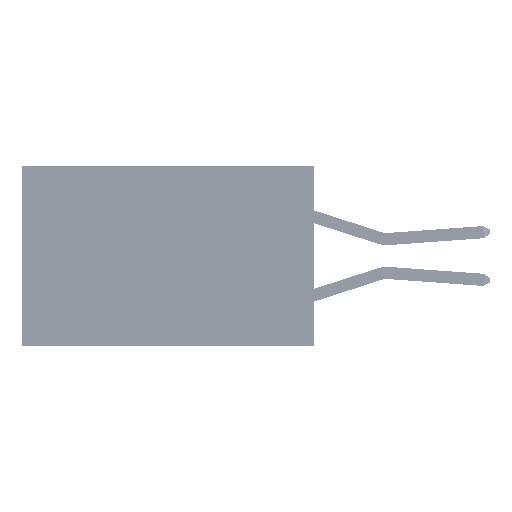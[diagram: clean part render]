
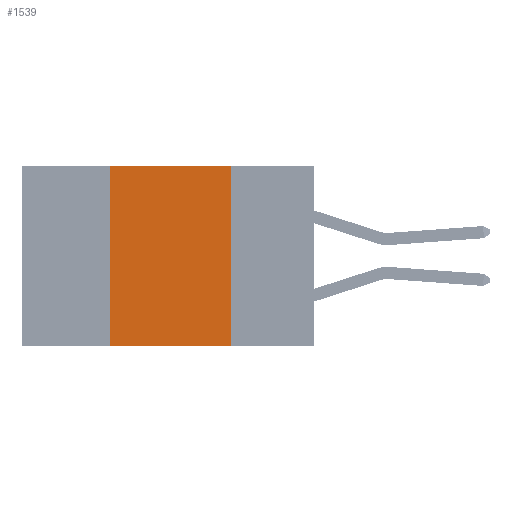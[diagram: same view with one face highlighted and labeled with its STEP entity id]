
A CAD part, left-side view. The second image highlights one B-rep face of the part: STEP entity #1539.
In plain terms, the highlighted planar face has unit normal (-1, 0, 0).
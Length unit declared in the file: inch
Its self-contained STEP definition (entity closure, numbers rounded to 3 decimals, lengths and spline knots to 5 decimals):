
#445 = CARTESIAN_POINT ( 'NONE',  ( 0., 0.42, -0.37 ) ) ;
#986 = DIRECTION ( 'NONE',  ( 0., 0., -1. ) ) ;
#1539 = ADVANCED_FACE ( 'NONE', ( #30907 ), #30218, .F. ) ;
#2058 = DIRECTION ( 'NONE',  ( 0., 0., -1. ) ) ;
#2326 = EDGE_CURVE ( 'NONE', #33802, #17893, #8206, .T. ) ;
#2948 = ORIENTED_EDGE ( 'NONE', *, *, #32629, .T. ) ;
#3927 = EDGE_LOOP ( 'NONE', ( #23682, #7659, #36213, #2948 ) ) ;
#5360 = LINE ( 'NONE', #33270, #23495 ) ;
#5584 = VECTOR ( 'NONE', #986, 39.37008 ) ;
#6009 = CARTESIAN_POINT ( 'NONE',  ( 0., 0.6, 0. ) ) ;
#6398 = VECTOR ( 'NONE', #20440, 39.37008 ) ;
#7060 = CARTESIAN_POINT ( 'NONE',  ( 0., 0.17, -0.37 ) ) ;
#7659 = ORIENTED_EDGE ( 'NONE', *, *, #41234, .F. ) ;
#8206 = LINE ( 'NONE', #43812, #5584 ) ;
#10143 = LINE ( 'NONE', #28269, #23420 ) ;
#10599 = DIRECTION ( 'NONE',  ( 0., 0., 1. ) ) ;
#12157 = VERTEX_POINT ( 'NONE', #445 ) ;
#16068 = DIRECTION ( 'NONE',  ( 0., -1., 0. ) ) ;
#17893 = VERTEX_POINT ( 'NONE', #7060 ) ;
#20440 = DIRECTION ( 'NONE',  ( 0., -1., 0. ) ) ;
#23420 = VECTOR ( 'NONE', #10599, 39.37008 ) ;
#23495 = VECTOR ( 'NONE', #16068, 39.37008 ) ;
#23682 = ORIENTED_EDGE ( 'NONE', *, *, #2326, .F. ) ;
#24752 = CARTESIAN_POINT ( 'NONE',  ( 0., 0.17, 0. ) ) ;
#26063 = AXIS2_PLACEMENT_3D ( 'NONE', #6009, #34383, #2058 ) ;
#28269 = CARTESIAN_POINT ( 'NONE',  ( 0., 0.42, 0. ) ) ;
#30218 = PLANE ( 'NONE',  #26063 ) ;
#30907 = FACE_OUTER_BOUND ( 'NONE', #3927, .T. ) ;
#32629 = EDGE_CURVE ( 'NONE', #12157, #17893, #5360, .T. ) ;
#33270 = CARTESIAN_POINT ( 'NONE',  ( 0., 0.6, -0.37 ) ) ;
#33723 = CARTESIAN_POINT ( 'NONE',  ( 0., 0.42, 0. ) ) ;
#33802 = VERTEX_POINT ( 'NONE', #24752 ) ;
#34383 = DIRECTION ( 'NONE',  ( 1., 0., 0. ) ) ;
#36213 = ORIENTED_EDGE ( 'NONE', *, *, #40194, .F. ) ;
#40194 = EDGE_CURVE ( 'NONE', #12157, #41099, #10143, .T. ) ;
#41099 = VERTEX_POINT ( 'NONE', #33723 ) ;
#41234 = EDGE_CURVE ( 'NONE', #41099, #33802, #41863, .T. ) ;
#41863 = LINE ( 'NONE', #45125, #6398 ) ;
#43812 = CARTESIAN_POINT ( 'NONE',  ( 0., 0.17, 0. ) ) ;
#45125 = CARTESIAN_POINT ( 'NONE',  ( 0., 0.6, 0. ) ) ;
